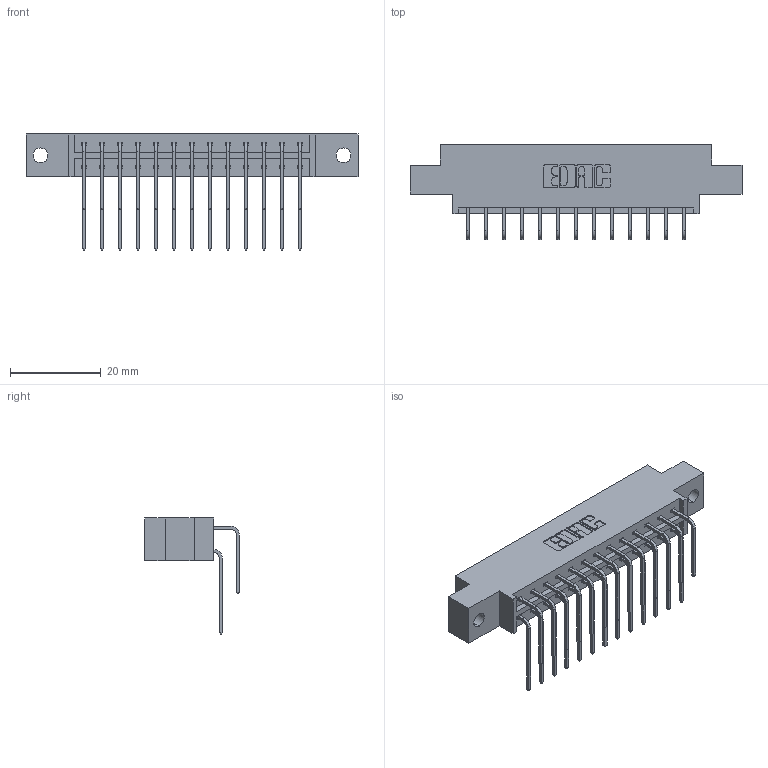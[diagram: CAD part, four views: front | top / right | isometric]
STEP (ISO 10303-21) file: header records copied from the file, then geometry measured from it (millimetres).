
FILE_DESCRIPTION (( 'STEP AP203' ), '1' );
FILE_NAME ('833-026-559-802.STEP', '2020-06-02T05:54:38', ( '' ), ( '' ), 'SwSTEP 2.0', 'SolidWorks 2020', '' );
FILE_SCHEMA (( 'CONFIG_CONTROL_DESIGN' ));
Length unit declared in the file: inch
Products named in the file (4): 345-292-001_559 Tail - 2; 833 Part_Offset - .128 Dia; 345-292-001_558 559 Tail - 1; 833-026-559-802
Assembly tree (27 placements, depth 2):
  833-026-559-802
    833 Part_Offset - .128 Dia
    345-292-001_558 559 Tail - 1  x13
    345-292-001_559 Tail - 2  x13
Bounding box: 73.05 x 20.9 x 25.53 mm (x, y, z)
Volume: 7072.3 mm3; surface area: 8744.2 mm2
Topology: 27 solids, 27 shells, 1522 faces, 4509 edges, 2970 vertices
Faces by surface type: plane 1062, cylinder 460
Entity records: 14033 total; most frequent: CARTESIAN_POINT 2413, ORIENTED_EDGE 2298, DIRECTION 2093, EDGE_CURVE 1149, VECTOR 981, LINE 981, VERTEX_POINT 762, AXIS2_PLACEMENT_3D 556
